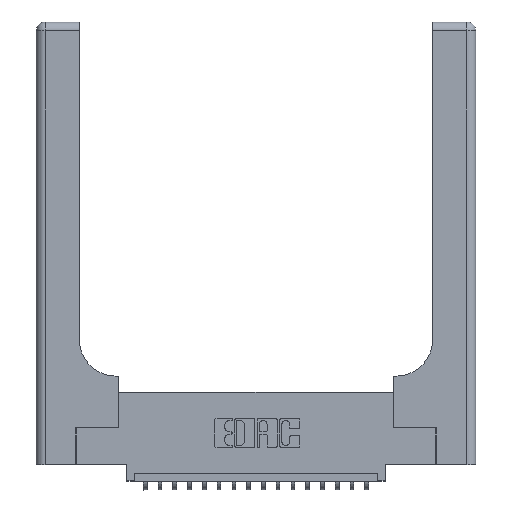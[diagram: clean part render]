
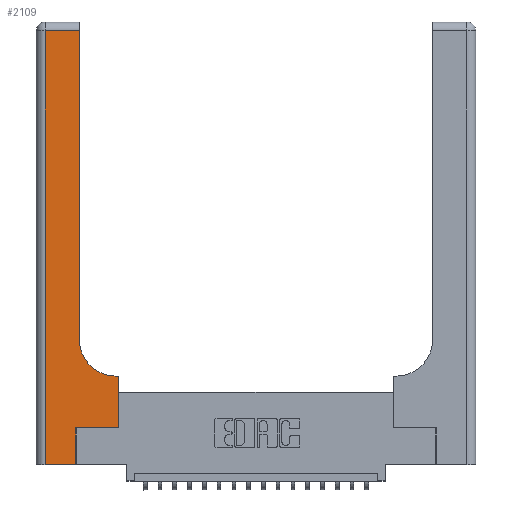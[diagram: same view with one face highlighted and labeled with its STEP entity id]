
A CAD part, top view. The second image highlights one B-rep face of the part: STEP entity #2109.
In plain terms, the highlighted planar face has unit normal (0, 0, 1).
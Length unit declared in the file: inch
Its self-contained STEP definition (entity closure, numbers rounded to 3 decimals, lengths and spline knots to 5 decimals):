
#65 = VECTOR ( 'NONE', #17012, 39.37008 ) ;
#189 = CARTESIAN_POINT ( 'NONE',  ( 0.269, 0., 0.37 ) ) ;
#228 = LINE ( 'NONE', #20422, #6301 ) ;
#492 = DIRECTION ( 'NONE',  ( 1., 0., 0. ) ) ;
#630 = DIRECTION ( 'NONE',  ( 0., 0., -1. ) ) ;
#734 = VERTEX_POINT ( 'NONE', #9753 ) ;
#1692 = ORIENTED_EDGE ( 'NONE', *, *, #11670, .T. ) ;
#2088 = EDGE_CURVE ( 'NONE', #20759, #734, #10711, .T. ) ;
#2109 = ADVANCED_FACE ( 'NONE', ( #11239 ), #13672, .F. ) ;
#2197 = DIRECTION ( 'NONE',  ( 0., 1., 0. ) ) ;
#2592 = CARTESIAN_POINT ( 'NONE',  ( 0., 0., 0.37 ) ) ;
#2894 = VERTEX_POINT ( 'NONE', #7881 ) ;
#3299 = CARTESIAN_POINT ( 'NONE',  ( 0.06, 2.94, 0.37 ) ) ;
#3422 = VECTOR ( 'NONE', #15218, 39.37008 ) ;
#3510 = VERTEX_POINT ( 'NONE', #4666 ) ;
#4049 = VECTOR ( 'NONE', #18941, 39.37008 ) ;
#4062 = DIRECTION ( 'NONE',  ( 0., 0., -1. ) ) ;
#4219 = ORIENTED_EDGE ( 'NONE', *, *, #6025, .T. ) ;
#4291 = LINE ( 'NONE', #12673, #4049 ) ;
#4324 = EDGE_LOOP ( 'NONE', ( #14486, #13055, #1692, #10650, #13433, #6380, #4354, #4219, #9063 ) ) ;
#4349 = LINE ( 'NONE', #7544, #65 ) ;
#4354 = ORIENTED_EDGE ( 'NONE', *, *, #2088, .T. ) ;
#4666 = CARTESIAN_POINT ( 'NONE',  ( 0.2915, 0.85, 0.37 ) ) ;
#5087 = AXIS2_PLACEMENT_3D ( 'NONE', #18304, #4062, #10384 ) ;
#5523 = VECTOR ( 'NONE', #18657, 39.37008 ) ;
#5543 = LINE ( 'NONE', #12957, #7053 ) ;
#6025 = EDGE_CURVE ( 'NONE', #734, #14950, #5543, .T. ) ;
#6078 = DIRECTION ( 'NONE',  ( 1., 0., 0. ) ) ;
#6208 = EDGE_CURVE ( 'NONE', #18758, #20759, #228, .T. ) ;
#6216 = EDGE_CURVE ( 'NONE', #2894, #18758, #14633, .T. ) ;
#6301 = VECTOR ( 'NONE', #6078, 39.37008 ) ;
#6380 = ORIENTED_EDGE ( 'NONE', *, *, #6208, .T. ) ;
#7053 = VECTOR ( 'NONE', #12748, 39.37008 ) ;
#7544 = CARTESIAN_POINT ( 'NONE',  ( 0.06, 3., 0.37 ) ) ;
#7881 = CARTESIAN_POINT ( 'NONE',  ( 0.269, 0., 0.37 ) ) ;
#8445 = CARTESIAN_POINT ( 'NONE',  ( 0.2915, 2.94, 0.37 ) ) ;
#8645 = VERTEX_POINT ( 'NONE', #20854 ) ;
#8821 = CARTESIAN_POINT ( 'NONE',  ( 0.269, 0.25, 0.37 ) ) ;
#9063 = ORIENTED_EDGE ( 'NONE', *, *, #12947, .T. ) ;
#9535 = LINE ( 'NONE', #2592, #11039 ) ;
#9592 = CIRCLE ( 'NONE', #17693, 0.25 ) ;
#9753 = CARTESIAN_POINT ( 'NONE',  ( 0.5585, 0.6, 0.37 ) ) ;
#10269 = CARTESIAN_POINT ( 'NONE',  ( 0.5415, 0.85, 0.37 ) ) ;
#10384 = DIRECTION ( 'NONE',  ( -1., 0., 0. ) ) ;
#10650 = ORIENTED_EDGE ( 'NONE', *, *, #17697, .T. ) ;
#10711 = LINE ( 'NONE', #20072, #3422 ) ;
#11039 = VECTOR ( 'NONE', #13882, 39.37008 ) ;
#11239 = FACE_OUTER_BOUND ( 'NONE', #4324, .T. ) ;
#11638 = CARTESIAN_POINT ( 'NONE',  ( 0.5585, 0.25, 0.37 ) ) ;
#11670 = EDGE_CURVE ( 'NONE', #20205, #8645, #4349, .T. ) ;
#12673 = CARTESIAN_POINT ( 'NONE',  ( 0., 2.94, 0.37 ) ) ;
#12748 = DIRECTION ( 'NONE',  ( -1., 0., 0. ) ) ;
#12947 = EDGE_CURVE ( 'NONE', #14950, #3510, #9592, .T. ) ;
#12957 = CARTESIAN_POINT ( 'NONE',  ( 0.2915, 0.6, 0.37 ) ) ;
#13055 = ORIENTED_EDGE ( 'NONE', *, *, #16283, .T. ) ;
#13433 = ORIENTED_EDGE ( 'NONE', *, *, #6216, .T. ) ;
#13672 = PLANE ( 'NONE',  #5087 ) ;
#13882 = DIRECTION ( 'NONE',  ( 1., 0., 0. ) ) ;
#14486 = ORIENTED_EDGE ( 'NONE', *, *, #16569, .T. ) ;
#14633 = LINE ( 'NONE', #189, #5523 ) ;
#14866 = VERTEX_POINT ( 'NONE', #8445 ) ;
#14950 = VERTEX_POINT ( 'NONE', #20541 ) ;
#15218 = DIRECTION ( 'NONE',  ( 0., 1., 0. ) ) ;
#16283 = EDGE_CURVE ( 'NONE', #14866, #20205, #4291, .T. ) ;
#16569 = EDGE_CURVE ( 'NONE', #3510, #14866, #20463, .T. ) ;
#17012 = DIRECTION ( 'NONE',  ( 0., -1., 0. ) ) ;
#17693 = AXIS2_PLACEMENT_3D ( 'NONE', #10269, #630, #492 ) ;
#17697 = EDGE_CURVE ( 'NONE', #8645, #2894, #9535, .T. ) ;
#17920 = VECTOR ( 'NONE', #2197, 39.37008 ) ;
#18304 = CARTESIAN_POINT ( 'NONE',  ( 0., 3., 0.37 ) ) ;
#18657 = DIRECTION ( 'NONE',  ( 0., 1., 0. ) ) ;
#18758 = VERTEX_POINT ( 'NONE', #8821 ) ;
#18941 = DIRECTION ( 'NONE',  ( -1., 0., 0. ) ) ;
#19558 = CARTESIAN_POINT ( 'NONE',  ( 0.2915, 3., 0.37 ) ) ;
#20072 = CARTESIAN_POINT ( 'NONE',  ( 0.5585, 0.25, 0.37 ) ) ;
#20205 = VERTEX_POINT ( 'NONE', #3299 ) ;
#20422 = CARTESIAN_POINT ( 'NONE',  ( 0.269, 0.25, 0.37 ) ) ;
#20463 = LINE ( 'NONE', #19558, #17920 ) ;
#20541 = CARTESIAN_POINT ( 'NONE',  ( 0.5415, 0.6, 0.37 ) ) ;
#20759 = VERTEX_POINT ( 'NONE', #11638 ) ;
#20854 = CARTESIAN_POINT ( 'NONE',  ( 0.06, 0., 0.37 ) ) ;
